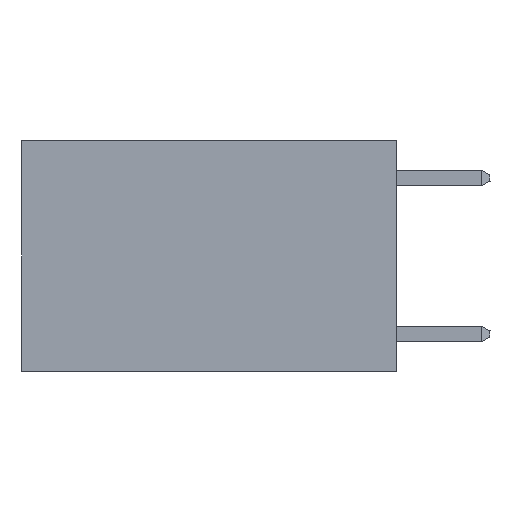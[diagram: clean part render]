
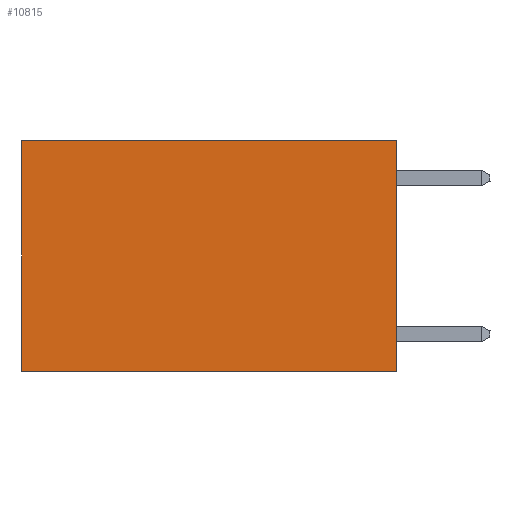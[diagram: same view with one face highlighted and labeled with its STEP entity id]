
A CAD part, left-side view. The second image highlights one B-rep face of the part: STEP entity #10815.
In plain terms, the highlighted planar face has unit normal (-1, 0, 0).
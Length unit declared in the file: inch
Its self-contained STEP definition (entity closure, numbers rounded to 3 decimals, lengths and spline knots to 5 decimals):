
#290 = LINE ( 'NONE', #5933, #6470 ) ;
#305 = CARTESIAN_POINT ( 'NONE',  ( 0.2625, 0., 0. ) ) ;
#343 = CARTESIAN_POINT ( 'NONE',  ( 0.2625, 0., -0.37 ) ) ;
#830 = CARTESIAN_POINT ( 'NONE',  ( 0.2625, 0.6, 0. ) ) ;
#991 = LINE ( 'NONE', #6444, #4442 ) ;
#1046 = LINE ( 'NONE', #5359, #8737 ) ;
#1060 = DIRECTION ( 'NONE',  ( 0., 0., -1. ) ) ;
#1096 = DIRECTION ( 'NONE',  ( 0., 1., 0. ) ) ;
#1518 = VECTOR ( 'NONE', #8038, 39.37008 ) ;
#2078 = LINE ( 'NONE', #830, #1518 ) ;
#2838 = PLANE ( 'NONE',  #3475 ) ;
#3345 = EDGE_CURVE ( 'NONE', #7518, #4161, #1046, .T. ) ;
#3475 = AXIS2_PLACEMENT_3D ( 'NONE', #7221, #8183, #1060 ) ;
#4061 = DIRECTION ( 'NONE',  ( 0., 1., 0. ) ) ;
#4161 = VERTEX_POINT ( 'NONE', #343 ) ;
#4438 = VERTEX_POINT ( 'NONE', #8215 ) ;
#4442 = VECTOR ( 'NONE', #1096, 39.37008 ) ;
#4752 = ORIENTED_EDGE ( 'NONE', *, *, #6421, .T. ) ;
#5359 = CARTESIAN_POINT ( 'NONE',  ( 0.2625, 0., 0. ) ) ;
#5681 = VERTEX_POINT ( 'NONE', #6618 ) ;
#5933 = CARTESIAN_POINT ( 'NONE',  ( 0.2625, 0., 0. ) ) ;
#6421 = EDGE_CURVE ( 'NONE', #7518, #4438, #290, .T. ) ;
#6444 = CARTESIAN_POINT ( 'NONE',  ( 0.2625, 0., -0.37 ) ) ;
#6470 = VECTOR ( 'NONE', #4061, 39.37008 ) ;
#6537 = ORIENTED_EDGE ( 'NONE', *, *, #8329, .T. ) ;
#6618 = CARTESIAN_POINT ( 'NONE',  ( 0.2625, 0.6, -0.37 ) ) ;
#7221 = CARTESIAN_POINT ( 'NONE',  ( 0.2625, 0., 0. ) ) ;
#7315 = ORIENTED_EDGE ( 'NONE', *, *, #8146, .F. ) ;
#7518 = VERTEX_POINT ( 'NONE', #305 ) ;
#8038 = DIRECTION ( 'NONE',  ( 0., 0., -1. ) ) ;
#8073 = FACE_OUTER_BOUND ( 'NONE', #8145, .T. ) ;
#8140 = DIRECTION ( 'NONE',  ( 0., 0., -1. ) ) ;
#8145 = EDGE_LOOP ( 'NONE', ( #6537, #7315, #9089, #4752 ) ) ;
#8146 = EDGE_CURVE ( 'NONE', #4161, #5681, #991, .T. ) ;
#8183 = DIRECTION ( 'NONE',  ( 1., 0., 0. ) ) ;
#8215 = CARTESIAN_POINT ( 'NONE',  ( 0.2625, 0.6, 0. ) ) ;
#8329 = EDGE_CURVE ( 'NONE', #4438, #5681, #2078, .T. ) ;
#8737 = VECTOR ( 'NONE', #8140, 39.37008 ) ;
#9089 = ORIENTED_EDGE ( 'NONE', *, *, #3345, .F. ) ;
#10815 = ADVANCED_FACE ( 'NONE', ( #8073 ), #2838, .F. ) ;
